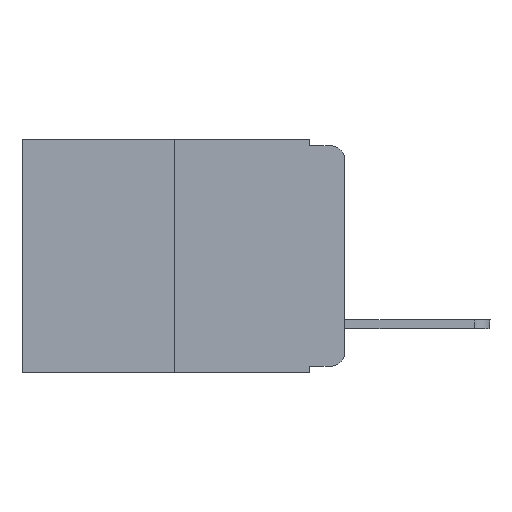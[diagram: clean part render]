
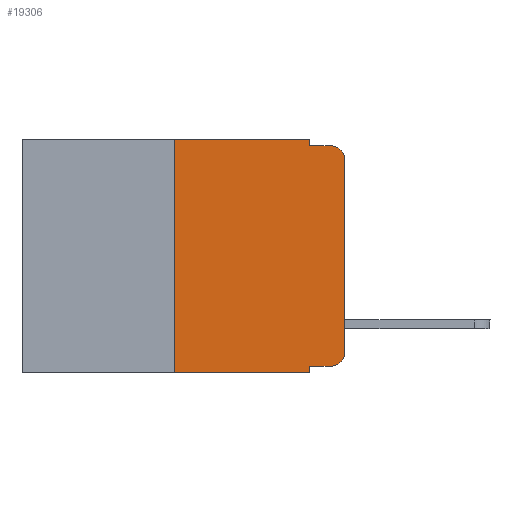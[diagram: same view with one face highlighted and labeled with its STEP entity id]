
A CAD part, left-side view. The second image highlights one B-rep face of the part: STEP entity #19306.
In plain terms, the highlighted planar face has unit normal (-1, 0, 0).
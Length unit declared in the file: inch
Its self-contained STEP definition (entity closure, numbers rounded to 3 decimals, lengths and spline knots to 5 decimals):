
#4 = LINE ( 'NONE', #5033, #9556 ) ;
#380 = AXIS2_PLACEMENT_3D ( 'NONE', #3586, #5579, #15713 ) ;
#510 = LINE ( 'NONE', #20902, #20681 ) ;
#838 = PLANE ( 'NONE',  #18047 ) ;
#859 = ORIENTED_EDGE ( 'NONE', *, *, #4934, .F. ) ;
#1155 = EDGE_CURVE ( 'NONE', #2340, #17844, #7690, .T. ) ;
#1700 = VERTEX_POINT ( 'NONE', #12807 ) ;
#1720 = EDGE_CURVE ( 'NONE', #16820, #21128, #21398, .T. ) ;
#1721 = CARTESIAN_POINT ( 'NONE',  ( 0., 0.051, -0.01 ) ) ;
#2129 = CARTESIAN_POINT ( 'NONE',  ( 0., 0.02, -0.01 ) ) ;
#2333 = DIRECTION ( 'NONE',  ( 0., 0., -1. ) ) ;
#2340 = VERTEX_POINT ( 'NONE', #8842 ) ;
#2629 = ORIENTED_EDGE ( 'NONE', *, *, #15072, .F. ) ;
#2788 = CIRCLE ( 'NONE', #15232, 0.02 ) ;
#3420 = CARTESIAN_POINT ( 'NONE',  ( 0., 0., -0.313 ) ) ;
#3543 = EDGE_CURVE ( 'NONE', #16820, #2340, #510, .T. ) ;
#3586 = CARTESIAN_POINT ( 'NONE',  ( 0., 0.02, -0.03 ) ) ;
#3899 = EDGE_LOOP ( 'NONE', ( #6536, #9153, #21095, #859, #6055, #17183, #6269, #2629, #19262, #17849 ) ) ;
#4506 = EDGE_CURVE ( 'NONE', #7650, #1700, #7587, .T. ) ;
#4801 = EDGE_CURVE ( 'NONE', #20871, #12778, #4, .T. ) ;
#4860 = VECTOR ( 'NONE', #14588, 39.37008 ) ;
#4934 = EDGE_CURVE ( 'NONE', #17844, #20871, #17487, .T. ) ;
#5033 = CARTESIAN_POINT ( 'NONE',  ( 0., 0.051, -0.01 ) ) ;
#5579 = DIRECTION ( 'NONE',  ( -1., 0., 0. ) ) ;
#5643 = DIRECTION ( 'NONE',  ( 0., 0., 1. ) ) ;
#5752 = FACE_OUTER_BOUND ( 'NONE', #3899, .T. ) ;
#6028 = CARTESIAN_POINT ( 'NONE',  ( 0., 0.473, 0. ) ) ;
#6055 = ORIENTED_EDGE ( 'NONE', *, *, #1155, .F. ) ;
#6269 = ORIENTED_EDGE ( 'NONE', *, *, #1720, .T. ) ;
#6536 = ORIENTED_EDGE ( 'NONE', *, *, #4506, .T. ) ;
#6613 = EDGE_CURVE ( 'NONE', #6676, #7650, #2788, .T. ) ;
#6676 = VERTEX_POINT ( 'NONE', #14594 ) ;
#7523 = DIRECTION ( 'NONE',  ( 1., 0., 0. ) ) ;
#7532 = EDGE_CURVE ( 'NONE', #10245, #6676, #16113, .T. ) ;
#7534 = DIRECTION ( 'NONE',  ( 0., -1., 0. ) ) ;
#7587 = LINE ( 'NONE', #14376, #19162 ) ;
#7633 = CARTESIAN_POINT ( 'NONE',  ( 0., 0.473, 0. ) ) ;
#7650 = VERTEX_POINT ( 'NONE', #3420 ) ;
#7690 = LINE ( 'NONE', #6028, #4860 ) ;
#8250 = VECTOR ( 'NONE', #19202, 39.37008 ) ;
#8842 = CARTESIAN_POINT ( 'NONE',  ( 0., 0.25, 0. ) ) ;
#9153 = ORIENTED_EDGE ( 'NONE', *, *, #14273, .T. ) ;
#9287 = VECTOR ( 'NONE', #7534, 39.37008 ) ;
#9556 = VECTOR ( 'NONE', #20397, 39.37008 ) ;
#10245 = VERTEX_POINT ( 'NONE', #10247 ) ;
#10247 = CARTESIAN_POINT ( 'NONE',  ( 0., 0.051, -0.333 ) ) ;
#10786 = CARTESIAN_POINT ( 'NONE',  ( 0., 0.051, 0. ) ) ;
#11490 = CARTESIAN_POINT ( 'NONE',  ( 0., 0.02, -0.313 ) ) ;
#12177 = CARTESIAN_POINT ( 'NONE',  ( 0., 0.051, 0. ) ) ;
#12778 = VERTEX_POINT ( 'NONE', #2129 ) ;
#12807 = CARTESIAN_POINT ( 'NONE',  ( 0., 0., -0.03 ) ) ;
#13060 = CARTESIAN_POINT ( 'NONE',  ( 0., 0.051, -0.343 ) ) ;
#14273 = EDGE_CURVE ( 'NONE', #1700, #12778, #18172, .T. ) ;
#14376 = CARTESIAN_POINT ( 'NONE',  ( 0., 0., 0. ) ) ;
#14481 = DIRECTION ( 'NONE',  ( 0., 0., -1. ) ) ;
#14588 = DIRECTION ( 'NONE',  ( 0., -1., 0. ) ) ;
#14589 = CARTESIAN_POINT ( 'NONE',  ( 0., 0.25, -0.343 ) ) ;
#14594 = CARTESIAN_POINT ( 'NONE',  ( 0., 0.02, -0.333 ) ) ;
#15072 = EDGE_CURVE ( 'NONE', #10245, #21128, #17197, .T. ) ;
#15232 = AXIS2_PLACEMENT_3D ( 'NONE', #11490, #19628, #14481 ) ;
#15502 = VECTOR ( 'NONE', #17823, 39.37008 ) ;
#15713 = DIRECTION ( 'NONE',  ( 0., 0., -1. ) ) ;
#16113 = LINE ( 'NONE', #19572, #9287 ) ;
#16465 = CARTESIAN_POINT ( 'NONE',  ( 0., 0.051, 0. ) ) ;
#16820 = VERTEX_POINT ( 'NONE', #14589 ) ;
#17183 = ORIENTED_EDGE ( 'NONE', *, *, #3543, .F. ) ;
#17197 = LINE ( 'NONE', #12177, #8250 ) ;
#17447 = DIRECTION ( 'NONE',  ( 0., 0., -1. ) ) ;
#17487 = LINE ( 'NONE', #10786, #20243 ) ;
#17823 = DIRECTION ( 'NONE',  ( 0., -1., 0. ) ) ;
#17844 = VERTEX_POINT ( 'NONE', #16465 ) ;
#17849 = ORIENTED_EDGE ( 'NONE', *, *, #6613, .T. ) ;
#18047 = AXIS2_PLACEMENT_3D ( 'NONE', #7633, #7523, #17447 ) ;
#18172 = CIRCLE ( 'NONE', #380, 0.02 ) ;
#19162 = VECTOR ( 'NONE', #21179, 39.37008 ) ;
#19202 = DIRECTION ( 'NONE',  ( 0., 0., -1. ) ) ;
#19262 = ORIENTED_EDGE ( 'NONE', *, *, #7532, .T. ) ;
#19306 = ADVANCED_FACE ( 'NONE', ( #5752 ), #838, .F. ) ;
#19572 = CARTESIAN_POINT ( 'NONE',  ( 0., 0.051, -0.333 ) ) ;
#19628 = DIRECTION ( 'NONE',  ( -1., 0., 0. ) ) ;
#20243 = VECTOR ( 'NONE', #2333, 39.37008 ) ;
#20397 = DIRECTION ( 'NONE',  ( 0., -1., 0. ) ) ;
#20681 = VECTOR ( 'NONE', #5643, 39.37008 ) ;
#20871 = VERTEX_POINT ( 'NONE', #1721 ) ;
#20902 = CARTESIAN_POINT ( 'NONE',  ( 0., 0.25, 0. ) ) ;
#21095 = ORIENTED_EDGE ( 'NONE', *, *, #4801, .F. ) ;
#21128 = VERTEX_POINT ( 'NONE', #13060 ) ;
#21179 = DIRECTION ( 'NONE',  ( 0., 0., 1. ) ) ;
#21398 = LINE ( 'NONE', #21617, #15502 ) ;
#21617 = CARTESIAN_POINT ( 'NONE',  ( 0., 0.473, -0.343 ) ) ;
